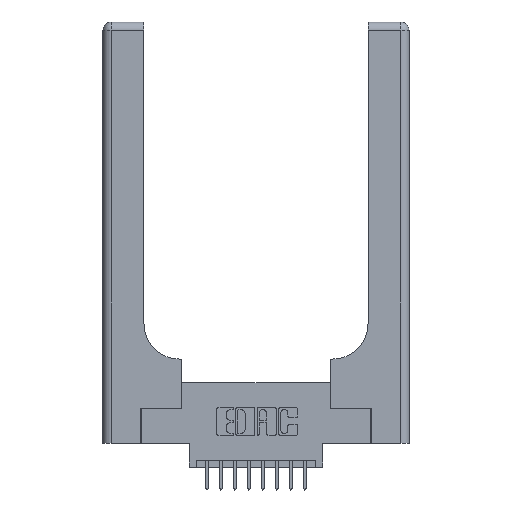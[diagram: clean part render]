
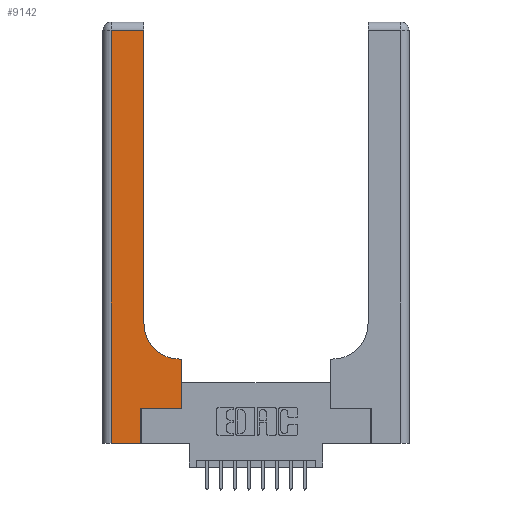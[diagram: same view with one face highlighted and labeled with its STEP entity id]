
A CAD part, top view. The second image highlights one B-rep face of the part: STEP entity #9142.
In plain terms, the highlighted planar face has unit normal (0, 0, 1).
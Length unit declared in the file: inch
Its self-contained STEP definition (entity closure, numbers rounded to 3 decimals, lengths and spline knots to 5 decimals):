
#37 = CARTESIAN_POINT ( 'NONE',  ( 0.2915, 3., 0.37 ) ) ;
#83 = DIRECTION ( 'NONE',  ( 1., 0., 0. ) ) ;
#149 = CIRCLE ( 'NONE', #529, 0.25 ) ;
#239 = CARTESIAN_POINT ( 'NONE',  ( 0.06, 3., 0.37 ) ) ;
#529 = AXIS2_PLACEMENT_3D ( 'NONE', #1630, #3009, #14216 ) ;
#748 = VERTEX_POINT ( 'NONE', #6399 ) ;
#779 = EDGE_CURVE ( 'NONE', #9036, #748, #8181, .T. ) ;
#1291 = VECTOR ( 'NONE', #9342, 39.37008 ) ;
#1399 = EDGE_CURVE ( 'NONE', #748, #3131, #4469, .T. ) ;
#1558 = PLANE ( 'NONE',  #3740 ) ;
#1630 = CARTESIAN_POINT ( 'NONE',  ( 0.5415, 0.85, 0.37 ) ) ;
#2531 = ORIENTED_EDGE ( 'NONE', *, *, #13026, .T. ) ;
#2803 = VECTOR ( 'NONE', #3925, 39.37008 ) ;
#2936 = ORIENTED_EDGE ( 'NONE', *, *, #11047, .T. ) ;
#3009 = DIRECTION ( 'NONE',  ( 0., 0., -1. ) ) ;
#3131 = VERTEX_POINT ( 'NONE', #10660 ) ;
#3155 = ORIENTED_EDGE ( 'NONE', *, *, #13693, .T. ) ;
#3161 = ORIENTED_EDGE ( 'NONE', *, *, #6381, .T. ) ;
#3385 = ORIENTED_EDGE ( 'NONE', *, *, #7005, .T. ) ;
#3740 = AXIS2_PLACEMENT_3D ( 'NONE', #5245, #11473, #12681 ) ;
#3925 = DIRECTION ( 'NONE',  ( -1., 0., 0. ) ) ;
#4257 = CARTESIAN_POINT ( 'NONE',  ( 0.06, 2.94, 0.37 ) ) ;
#4469 = LINE ( 'NONE', #15987, #8576 ) ;
#4477 = EDGE_CURVE ( 'NONE', #3131, #4889, #8468, .T. ) ;
#4592 = DIRECTION ( 'NONE',  ( 0., 1., 0. ) ) ;
#4640 = ORIENTED_EDGE ( 'NONE', *, *, #779, .T. ) ;
#4889 = VERTEX_POINT ( 'NONE', #9990 ) ;
#5224 = CARTESIAN_POINT ( 'NONE',  ( 0., 2.94, 0.37 ) ) ;
#5245 = CARTESIAN_POINT ( 'NONE',  ( 0., 3., 0.37 ) ) ;
#5520 = VERTEX_POINT ( 'NONE', #13463 ) ;
#5662 = VERTEX_POINT ( 'NONE', #10106 ) ;
#5745 = DIRECTION ( 'NONE',  ( -1., 0., 0. ) ) ;
#5757 = LINE ( 'NONE', #239, #8312 ) ;
#6016 = CARTESIAN_POINT ( 'NONE',  ( 0.269, 0., 0.37 ) ) ;
#6308 = VECTOR ( 'NONE', #5745, 39.37008 ) ;
#6381 = EDGE_CURVE ( 'NONE', #7067, #5520, #13428, .T. ) ;
#6399 = CARTESIAN_POINT ( 'NONE',  ( 0.5585, 0.25, 0.37 ) ) ;
#6714 = VECTOR ( 'NONE', #13506, 39.37008 ) ;
#7005 = EDGE_CURVE ( 'NONE', #5520, #9036, #10066, .T. ) ;
#7067 = VERTEX_POINT ( 'NONE', #9334 ) ;
#8181 = LINE ( 'NONE', #12575, #15695 ) ;
#8312 = VECTOR ( 'NONE', #10132, 39.37008 ) ;
#8468 = LINE ( 'NONE', #13336, #6308 ) ;
#8576 = VECTOR ( 'NONE', #4592, 39.37008 ) ;
#9036 = VERTEX_POINT ( 'NONE', #11312 ) ;
#9142 = ADVANCED_FACE ( 'NONE', ( #9390 ), #1558, .F. ) ;
#9239 = VERTEX_POINT ( 'NONE', #4257 ) ;
#9334 = CARTESIAN_POINT ( 'NONE',  ( 0.06, 0., 0.37 ) ) ;
#9342 = DIRECTION ( 'NONE',  ( 1., 0., 0. ) ) ;
#9390 = FACE_OUTER_BOUND ( 'NONE', #10065, .T. ) ;
#9769 = CARTESIAN_POINT ( 'NONE',  ( 0.2915, 0.85, 0.37 ) ) ;
#9990 = CARTESIAN_POINT ( 'NONE',  ( 0.5415, 0.6, 0.37 ) ) ;
#10065 = EDGE_LOOP ( 'NONE', ( #15790, #3155, #2531, #3161, #3385, #4640, #16034, #12666, #2936 ) ) ;
#10066 = LINE ( 'NONE', #6016, #6714 ) ;
#10106 = CARTESIAN_POINT ( 'NONE',  ( 0.2915, 2.94, 0.37 ) ) ;
#10132 = DIRECTION ( 'NONE',  ( 0., -1., 0. ) ) ;
#10660 = CARTESIAN_POINT ( 'NONE',  ( 0.5585, 0.6, 0.37 ) ) ;
#11047 = EDGE_CURVE ( 'NONE', #4889, #14184, #149, .T. ) ;
#11258 = LINE ( 'NONE', #37, #15596 ) ;
#11312 = CARTESIAN_POINT ( 'NONE',  ( 0.269, 0.25, 0.37 ) ) ;
#11473 = DIRECTION ( 'NONE',  ( 0., 0., -1. ) ) ;
#11849 = LINE ( 'NONE', #5224, #2803 ) ;
#11904 = CARTESIAN_POINT ( 'NONE',  ( 0., 0., 0.37 ) ) ;
#12370 = DIRECTION ( 'NONE',  ( 0., 1., 0. ) ) ;
#12575 = CARTESIAN_POINT ( 'NONE',  ( 0.269, 0.25, 0.37 ) ) ;
#12666 = ORIENTED_EDGE ( 'NONE', *, *, #4477, .T. ) ;
#12681 = DIRECTION ( 'NONE',  ( -1., 0., 0. ) ) ;
#13026 = EDGE_CURVE ( 'NONE', #9239, #7067, #5757, .T. ) ;
#13336 = CARTESIAN_POINT ( 'NONE',  ( 0.2915, 0.6, 0.37 ) ) ;
#13428 = LINE ( 'NONE', #11904, #1291 ) ;
#13463 = CARTESIAN_POINT ( 'NONE',  ( 0.269, 0., 0.37 ) ) ;
#13506 = DIRECTION ( 'NONE',  ( 0., 1., 0. ) ) ;
#13639 = EDGE_CURVE ( 'NONE', #14184, #5662, #11258, .T. ) ;
#13693 = EDGE_CURVE ( 'NONE', #5662, #9239, #11849, .T. ) ;
#14184 = VERTEX_POINT ( 'NONE', #9769 ) ;
#14216 = DIRECTION ( 'NONE',  ( 1., 0., 0. ) ) ;
#15596 = VECTOR ( 'NONE', #12370, 39.37008 ) ;
#15695 = VECTOR ( 'NONE', #83, 39.37008 ) ;
#15790 = ORIENTED_EDGE ( 'NONE', *, *, #13639, .T. ) ;
#15987 = CARTESIAN_POINT ( 'NONE',  ( 0.5585, 0.25, 0.37 ) ) ;
#16034 = ORIENTED_EDGE ( 'NONE', *, *, #1399, .T. ) ;
